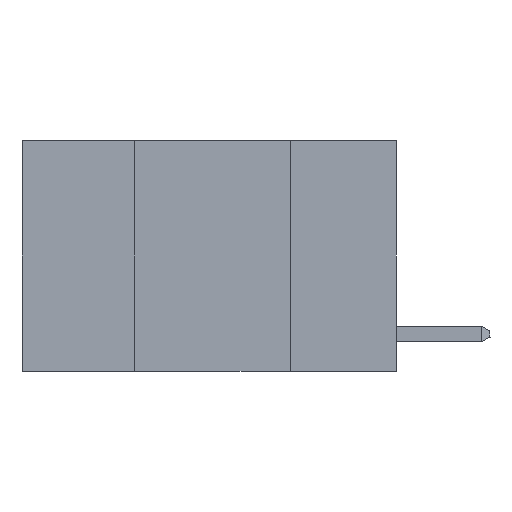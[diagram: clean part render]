
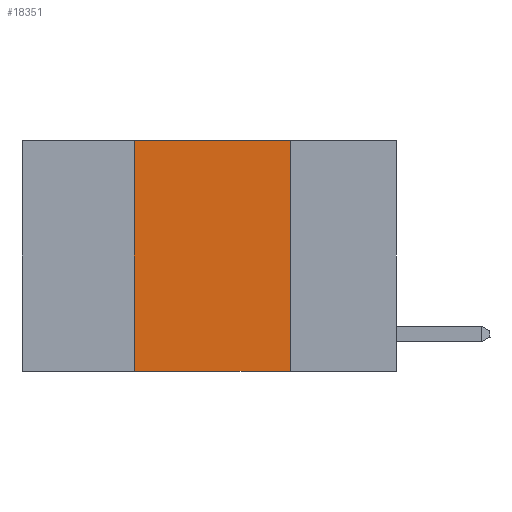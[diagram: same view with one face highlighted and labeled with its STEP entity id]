
A CAD part, left-side view. The second image highlights one B-rep face of the part: STEP entity #18351.
In plain terms, the highlighted planar face has unit normal (-1, 0, 0).
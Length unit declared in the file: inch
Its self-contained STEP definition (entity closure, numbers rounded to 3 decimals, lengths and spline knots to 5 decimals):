
#648 = VECTOR ( 'NONE', #5350, 39.37008 ) ;
#840 = DIRECTION ( 'NONE',  ( 0., 0., -1. ) ) ;
#974 = ORIENTED_EDGE ( 'NONE', *, *, #13781, .F. ) ;
#1635 = VERTEX_POINT ( 'NONE', #2255 ) ;
#1914 = VECTOR ( 'NONE', #3993, 39.37008 ) ;
#2255 = CARTESIAN_POINT ( 'NONE',  ( 0., 0.17, 0. ) ) ;
#3059 = CARTESIAN_POINT ( 'NONE',  ( 0., 0.6, 0. ) ) ;
#3900 = PLANE ( 'NONE',  #25541 ) ;
#3993 = DIRECTION ( 'NONE',  ( 0., -1., 0. ) ) ;
#5350 = DIRECTION ( 'NONE',  ( 0., -1., 0. ) ) ;
#6663 = LINE ( 'NONE', #27796, #23854 ) ;
#7077 = LINE ( 'NONE', #15543, #24981 ) ;
#7696 = EDGE_CURVE ( 'NONE', #28856, #11946, #7077, .T. ) ;
#8423 = ORIENTED_EDGE ( 'NONE', *, *, #18356, .T. ) ;
#8432 = CARTESIAN_POINT ( 'NONE',  ( 0., 0.6, 0. ) ) ;
#10705 = DIRECTION ( 'NONE',  ( 1., 0., 0. ) ) ;
#11946 = VERTEX_POINT ( 'NONE', #28698 ) ;
#13781 = EDGE_CURVE ( 'NONE', #1635, #20734, #6663, .T. ) ;
#15245 = EDGE_LOOP ( 'NONE', ( #974, #18381, #24939, #8423 ) ) ;
#15543 = CARTESIAN_POINT ( 'NONE',  ( 0., 0.42, 0. ) ) ;
#16043 = EDGE_CURVE ( 'NONE', #11946, #1635, #18740, .T. ) ;
#18351 = ADVANCED_FACE ( 'NONE', ( #25139 ), #3900, .F. ) ;
#18356 = EDGE_CURVE ( 'NONE', #28856, #20734, #19250, .T. ) ;
#18381 = ORIENTED_EDGE ( 'NONE', *, *, #16043, .F. ) ;
#18740 = LINE ( 'NONE', #3059, #648 ) ;
#19250 = LINE ( 'NONE', #28616, #1914 ) ;
#20036 = DIRECTION ( 'NONE',  ( 0., 0., 1. ) ) ;
#20734 = VERTEX_POINT ( 'NONE', #21669 ) ;
#21669 = CARTESIAN_POINT ( 'NONE',  ( 0., 0.17, -0.37 ) ) ;
#23854 = VECTOR ( 'NONE', #840, 39.37008 ) ;
#24939 = ORIENTED_EDGE ( 'NONE', *, *, #7696, .F. ) ;
#24981 = VECTOR ( 'NONE', #20036, 39.37008 ) ;
#25139 = FACE_OUTER_BOUND ( 'NONE', #15245, .T. ) ;
#25541 = AXIS2_PLACEMENT_3D ( 'NONE', #8432, #10705, #26372 ) ;
#26372 = DIRECTION ( 'NONE',  ( 0., 0., -1. ) ) ;
#27022 = CARTESIAN_POINT ( 'NONE',  ( 0., 0.42, -0.37 ) ) ;
#27796 = CARTESIAN_POINT ( 'NONE',  ( 0., 0.17, 0. ) ) ;
#28616 = CARTESIAN_POINT ( 'NONE',  ( 0., 0.6, -0.37 ) ) ;
#28698 = CARTESIAN_POINT ( 'NONE',  ( 0., 0.42, 0. ) ) ;
#28856 = VERTEX_POINT ( 'NONE', #27022 ) ;
